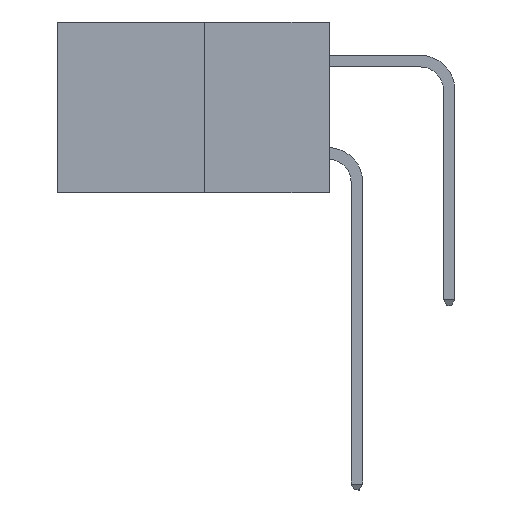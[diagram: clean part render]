
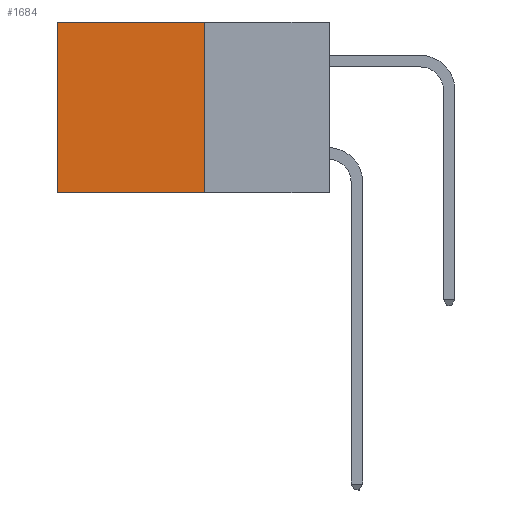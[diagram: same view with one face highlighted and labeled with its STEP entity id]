
A CAD part, left-side view. The second image highlights one B-rep face of the part: STEP entity #1684.
In plain terms, the highlighted planar face has unit normal (-1, 0, 0).
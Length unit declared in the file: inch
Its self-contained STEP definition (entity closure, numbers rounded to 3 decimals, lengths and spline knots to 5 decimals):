
#135 = DIRECTION ( 'NONE',  ( 0., 0., -1. ) ) ;
#838 = EDGE_LOOP ( 'NONE', ( #5521, #8170, #4576, #10565 ) ) ;
#1684 = ADVANCED_FACE ( 'NONE', ( #7838 ), #6924, .F. ) ;
#2014 = LINE ( 'NONE', #5722, #6388 ) ;
#3386 = VECTOR ( 'NONE', #3780, 39.37008 ) ;
#3764 = VERTEX_POINT ( 'NONE', #8025 ) ;
#3780 = DIRECTION ( 'NONE',  ( 0., 1., 0. ) ) ;
#3876 = CARTESIAN_POINT ( 'NONE',  ( 0.277, 0.59, 0. ) ) ;
#3939 = VERTEX_POINT ( 'NONE', #10850 ) ;
#4168 = EDGE_CURVE ( 'NONE', #8519, #3939, #8194, .T. ) ;
#4521 = EDGE_CURVE ( 'NONE', #4602, #3939, #5209, .T. ) ;
#4576 = ORIENTED_EDGE ( 'NONE', *, *, #10700, .F. ) ;
#4602 = VERTEX_POINT ( 'NONE', #3876 ) ;
#5209 = LINE ( 'NONE', #5481, #6953 ) ;
#5481 = CARTESIAN_POINT ( 'NONE',  ( 0.277, 0.59, -0.37 ) ) ;
#5492 = CARTESIAN_POINT ( 'NONE',  ( 0.277, 0.27, 0. ) ) ;
#5521 = ORIENTED_EDGE ( 'NONE', *, *, #4521, .T. ) ;
#5722 = CARTESIAN_POINT ( 'NONE',  ( 0.277, 0.27, -0.37 ) ) ;
#6388 = VECTOR ( 'NONE', #6581, 39.37008 ) ;
#6581 = DIRECTION ( 'NONE',  ( 0., 0., -1. ) ) ;
#6924 = PLANE ( 'NONE',  #10450 ) ;
#6953 = VECTOR ( 'NONE', #135, 39.37008 ) ;
#7262 = EDGE_CURVE ( 'NONE', #3764, #4602, #10575, .T. ) ;
#7348 = CARTESIAN_POINT ( 'NONE',  ( 0.277, 0.27, -0.37 ) ) ;
#7838 = FACE_OUTER_BOUND ( 'NONE', #838, .T. ) ;
#8025 = CARTESIAN_POINT ( 'NONE',  ( 0.277, 0.27, 0. ) ) ;
#8170 = ORIENTED_EDGE ( 'NONE', *, *, #4168, .F. ) ;
#8194 = LINE ( 'NONE', #10301, #10226 ) ;
#8241 = CARTESIAN_POINT ( 'NONE',  ( 0.277, 0.27, -0.37 ) ) ;
#8519 = VERTEX_POINT ( 'NONE', #7348 ) ;
#9420 = DIRECTION ( 'NONE',  ( 0., 1., 0. ) ) ;
#10226 = VECTOR ( 'NONE', #9420, 39.37008 ) ;
#10301 = CARTESIAN_POINT ( 'NONE',  ( 0.277, 0.27, -0.37 ) ) ;
#10450 = AXIS2_PLACEMENT_3D ( 'NONE', #8241, #11230, #10734 ) ;
#10565 = ORIENTED_EDGE ( 'NONE', *, *, #7262, .T. ) ;
#10575 = LINE ( 'NONE', #5492, #3386 ) ;
#10700 = EDGE_CURVE ( 'NONE', #3764, #8519, #2014, .T. ) ;
#10734 = DIRECTION ( 'NONE',  ( 0., 0., -1. ) ) ;
#10850 = CARTESIAN_POINT ( 'NONE',  ( 0.277, 0.59, -0.37 ) ) ;
#11230 = DIRECTION ( 'NONE',  ( 1., 0., 0. ) ) ;
